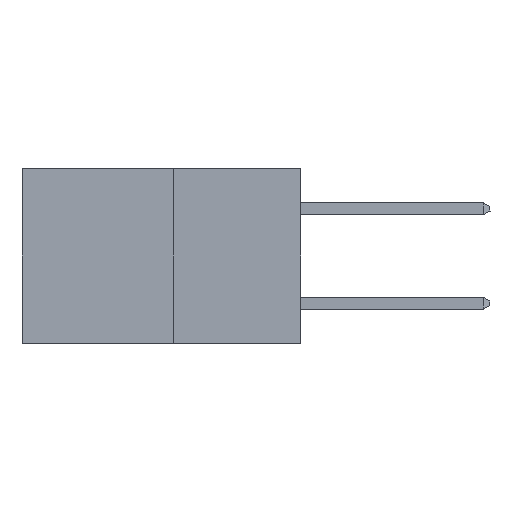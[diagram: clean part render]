
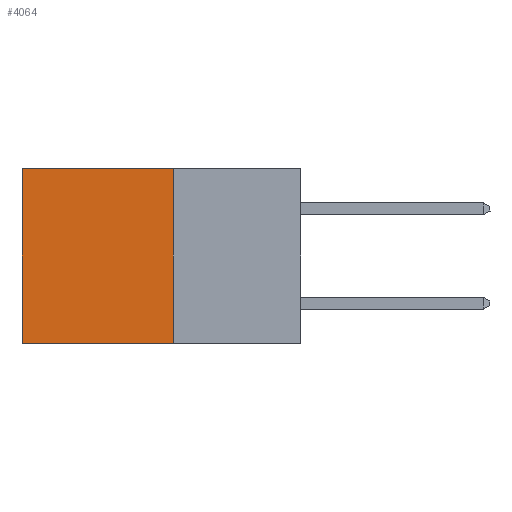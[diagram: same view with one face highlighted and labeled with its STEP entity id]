
A CAD part, left-side view. The second image highlights one B-rep face of the part: STEP entity #4064.
In plain terms, the highlighted planar face has unit normal (-1, 0, 0).
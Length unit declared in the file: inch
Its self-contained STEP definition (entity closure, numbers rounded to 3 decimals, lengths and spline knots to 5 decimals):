
#71 = DIRECTION ( 'NONE',  ( 0., 0., -1. ) ) ;
#545 = EDGE_CURVE ( 'NONE', #4245, #4189, #2378, .T. ) ;
#1866 = EDGE_CURVE ( 'NONE', #4189, #3279, #2570, .T. ) ;
#1867 = CARTESIAN_POINT ( 'NONE',  ( 0.277, 0.27, -0.37 ) ) ;
#2129 = LINE ( 'NONE', #15777, #5178 ) ;
#2378 = LINE ( 'NONE', #14702, #12718 ) ;
#2381 = EDGE_CURVE ( 'NONE', #4245, #14005, #2129, .T. ) ;
#2570 = LINE ( 'NONE', #14707, #15839 ) ;
#3279 = VERTEX_POINT ( 'NONE', #12150 ) ;
#3534 = EDGE_CURVE ( 'NONE', #14005, #3279, #11718, .T. ) ;
#3571 = ORIENTED_EDGE ( 'NONE', *, *, #2381, .F. ) ;
#4064 = ADVANCED_FACE ( 'NONE', ( #16417 ), #7261, .F. ) ;
#4189 = VERTEX_POINT ( 'NONE', #8428 ) ;
#4245 = VERTEX_POINT ( 'NONE', #16042 ) ;
#5178 = VECTOR ( 'NONE', #15849, 39.37008 ) ;
#7261 = PLANE ( 'NONE',  #13055 ) ;
#7311 = CARTESIAN_POINT ( 'NONE',  ( 0.277, 0.27, -0.37 ) ) ;
#7671 = CARTESIAN_POINT ( 'NONE',  ( 0.277, 0.27, -0.37 ) ) ;
#8428 = CARTESIAN_POINT ( 'NONE',  ( 0.277, 0.59, 0. ) ) ;
#9180 = EDGE_LOOP ( 'NONE', ( #13095, #16384, #3571, #14689 ) ) ;
#9354 = DIRECTION ( 'NONE',  ( 0., 0., -1. ) ) ;
#9432 = DIRECTION ( 'NONE',  ( 1., 0., 0. ) ) ;
#11718 = LINE ( 'NONE', #7311, #15128 ) ;
#12150 = CARTESIAN_POINT ( 'NONE',  ( 0.277, 0.59, -0.37 ) ) ;
#12718 = VECTOR ( 'NONE', #16170, 39.37008 ) ;
#13055 = AXIS2_PLACEMENT_3D ( 'NONE', #7671, #9432, #9354 ) ;
#13095 = ORIENTED_EDGE ( 'NONE', *, *, #1866, .T. ) ;
#14005 = VERTEX_POINT ( 'NONE', #1867 ) ;
#14689 = ORIENTED_EDGE ( 'NONE', *, *, #545, .T. ) ;
#14702 = CARTESIAN_POINT ( 'NONE',  ( 0.277, 0.27, 0. ) ) ;
#14707 = CARTESIAN_POINT ( 'NONE',  ( 0.277, 0.59, -0.37 ) ) ;
#15128 = VECTOR ( 'NONE', #16051, 39.37008 ) ;
#15777 = CARTESIAN_POINT ( 'NONE',  ( 0.277, 0.27, -0.37 ) ) ;
#15839 = VECTOR ( 'NONE', #71, 39.37008 ) ;
#15849 = DIRECTION ( 'NONE',  ( 0., 0., -1. ) ) ;
#16042 = CARTESIAN_POINT ( 'NONE',  ( 0.277, 0.27, 0. ) ) ;
#16051 = DIRECTION ( 'NONE',  ( 0., 1., 0. ) ) ;
#16170 = DIRECTION ( 'NONE',  ( 0., 1., 0. ) ) ;
#16384 = ORIENTED_EDGE ( 'NONE', *, *, #3534, .F. ) ;
#16417 = FACE_OUTER_BOUND ( 'NONE', #9180, .T. ) ;
